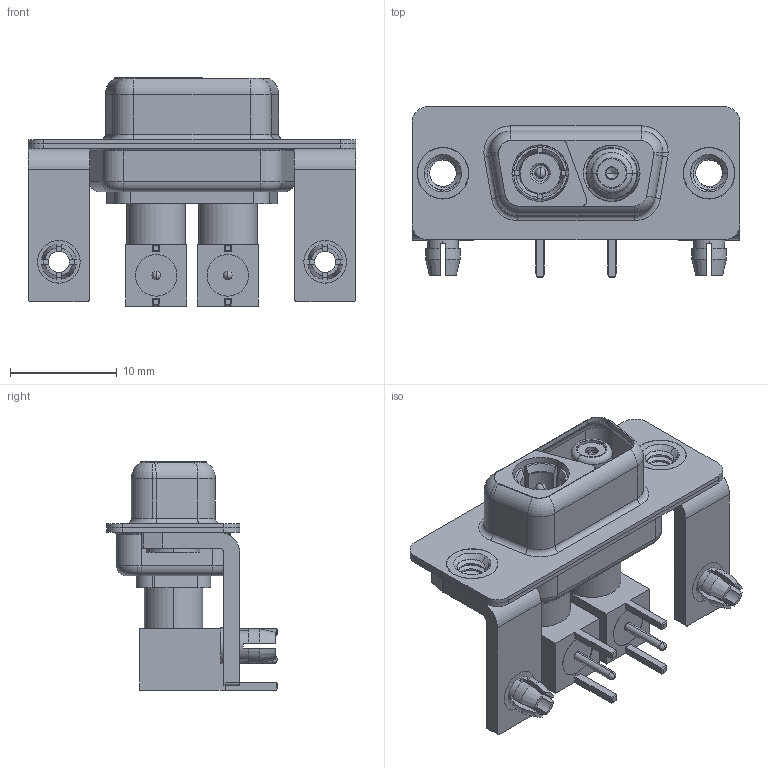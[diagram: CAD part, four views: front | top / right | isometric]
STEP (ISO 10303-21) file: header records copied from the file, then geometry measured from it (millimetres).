
FILE_DESCRIPTION (( 'STEP AP203' ), '1' );
FILE_NAME ('630-2WK2240-5TB.STEP', '2022-05-26T23:29:25', ( '' ), ( '' ), 'SwSTEP 2.0', 'SolidWorks 2020', '' );
FILE_SCHEMA (( 'CONFIG_CONTROL_DESIGN' ));
Length unit declared in the file: millimetre
Products named in the file (19): Co-Ax Plug_RA PC Tail; 630Combo Shell Rear_09 Contacts; Locking Collar; 630Combo Board Lock; 630Combo Threaded Rivet_B; RA Back Shell; Pin_RA; 630Combo Shell Front_09 Contacts; Socket_RA; Co-Ax Plug Assy_RA; Co-Ax Jack_RA PC Tail; Insulator RA Pin; 630Combo Stabilizer Bracket; Insulator Socket 2; Co-Ax Jack Assy_RA; Insulator Pin_Straight PC Tail; Insulator Socket; 630Combo Housing_2WK2; 630-2WK2240-5TB
Assembly tree (24 placements, depth 3):
  630-2WK2240-5TB
    630Combo Housing_2WK2
    630Combo Shell Front_09 Contacts
    630Combo Shell Rear_09 Contacts
    630Combo Threaded Rivet_B  x2
    630Combo Stabilizer Bracket  x2
    630Combo Board Lock  x2
    Co-Ax Plug Assy_RA
      Co-Ax Plug_RA PC Tail
      Insulator Pin_Straight PC Tail
      Pin_RA
      Locking Collar
      RA Back Shell
      Insulator RA Pin
    Co-Ax Jack Assy_RA
      Co-Ax Jack_RA PC Tail
      Insulator Socket
      Insulator Socket 2
      Locking Collar
      Socket_RA
      RA Back Shell
      Insulator RA Pin
Bounding box: 30.8 x 16 x 21.41 mm (x, y, z)
Volume: 2309.5 mm3; surface area: 6366.1 mm2
Topology: 22 solids, 22 shells, 730 faces, 1778 edges, 1119 vertices
Faces by surface type: cylinder 320, plane 259, torus 69, cone 68, bspline 8, sphere 6
Entity records: 20750 total; most frequent: CARTESIAN_POINT 4774, DIRECTION 3120, ORIENTED_EDGE 2744, EDGE_CURVE 1372, AXIS2_PLACEMENT_3D 1259, VERTEX_POINT 869, CIRCLE 659, EDGE_LOOP 653
